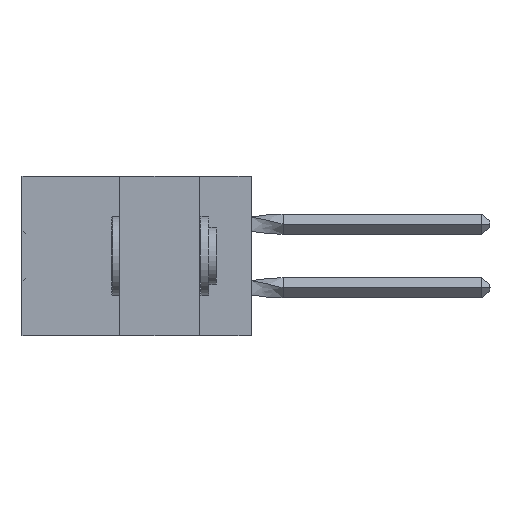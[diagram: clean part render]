
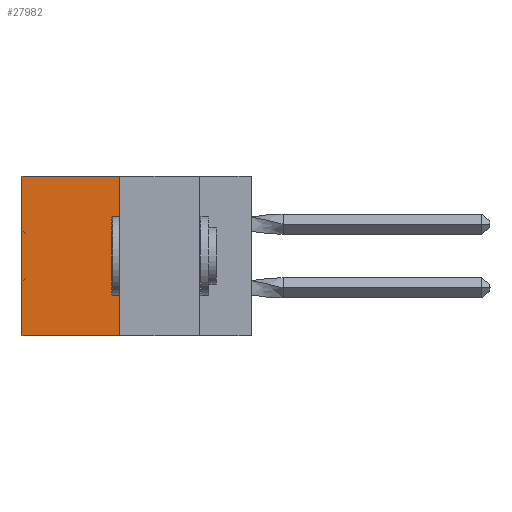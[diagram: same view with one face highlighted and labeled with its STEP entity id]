
A CAD part, left-side view. The second image highlights one B-rep face of the part: STEP entity #27982.
In plain terms, the highlighted planar face has unit normal (-1, 0, 0).
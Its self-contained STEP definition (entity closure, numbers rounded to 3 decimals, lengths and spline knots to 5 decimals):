
#197 = VERTEX_POINT ( 'NONE', #52741 ) ;
#777 = EDGE_CURVE ( 'NONE', #7615, #40959, #47508, .T. ) ;
#928 = DIRECTION ( 'NONE',  ( 0., 0., -1. ) ) ;
#2007 = CARTESIAN_POINT ( 'NONE',  ( 0.305, 0.413, 0. ) ) ;
#3601 = CARTESIAN_POINT ( 'NONE',  ( 0.305, 0.413, 0. ) ) ;
#3687 = CARTESIAN_POINT ( 'NONE',  ( 0.305, 0.413, -0.5 ) ) ;
#7615 = VERTEX_POINT ( 'NONE', #2007 ) ;
#9031 = EDGE_CURVE ( 'NONE', #197, #13418, #42977, .T. ) ;
#9338 = EDGE_LOOP ( 'NONE', ( #46517, #27417, #33806, #24617 ) ) ;
#13418 = VERTEX_POINT ( 'NONE', #35956 ) ;
#13648 = VECTOR ( 'NONE', #42796, 39.37008 ) ;
#16057 = FACE_OUTER_BOUND ( 'NONE', #9338, .T. ) ;
#16321 = VECTOR ( 'NONE', #52754, 39.37008 ) ;
#21499 = CARTESIAN_POINT ( 'NONE',  ( 0.305, 0.72, -0.5 ) ) ;
#24617 = ORIENTED_EDGE ( 'NONE', *, *, #777, .T. ) ;
#26058 = LINE ( 'NONE', #3687, #16321 ) ;
#26697 = PLANE ( 'NONE',  #38898 ) ;
#27417 = ORIENTED_EDGE ( 'NONE', *, *, #9031, .F. ) ;
#27982 = ADVANCED_FACE ( 'NONE', ( #16057 ), #26697, .F. ) ;
#29379 = CARTESIAN_POINT ( 'NONE',  ( 0.305, 0.72, 0. ) ) ;
#30216 = LINE ( 'NONE', #21499, #13648 ) ;
#31535 = VECTOR ( 'NONE', #53045, 39.37008 ) ;
#31948 = DIRECTION ( 'NONE',  ( 1., 0., 0. ) ) ;
#32568 = VECTOR ( 'NONE', #41182, 39.37008 ) ;
#33770 = EDGE_CURVE ( 'NONE', #7615, #197, #26058, .T. ) ;
#33806 = ORIENTED_EDGE ( 'NONE', *, *, #33770, .F. ) ;
#35956 = CARTESIAN_POINT ( 'NONE',  ( 0.305, 0.72, -0.5 ) ) ;
#38898 = AXIS2_PLACEMENT_3D ( 'NONE', #40082, #31948, #928 ) ;
#40082 = CARTESIAN_POINT ( 'NONE',  ( 0.305, 0.413, -0.5 ) ) ;
#40959 = VERTEX_POINT ( 'NONE', #29379 ) ;
#41182 = DIRECTION ( 'NONE',  ( 0., 1., 0. ) ) ;
#42796 = DIRECTION ( 'NONE',  ( 0., 0., -1. ) ) ;
#42977 = LINE ( 'NONE', #54532, #32568 ) ;
#45749 = EDGE_CURVE ( 'NONE', #40959, #13418, #30216, .T. ) ;
#46517 = ORIENTED_EDGE ( 'NONE', *, *, #45749, .T. ) ;
#47508 = LINE ( 'NONE', #3601, #31535 ) ;
#52741 = CARTESIAN_POINT ( 'NONE',  ( 0.305, 0.413, -0.5 ) ) ;
#52754 = DIRECTION ( 'NONE',  ( 0., 0., -1. ) ) ;
#53045 = DIRECTION ( 'NONE',  ( 0., 1., 0. ) ) ;
#54532 = CARTESIAN_POINT ( 'NONE',  ( 0.305, 0.413, -0.5 ) ) ;
